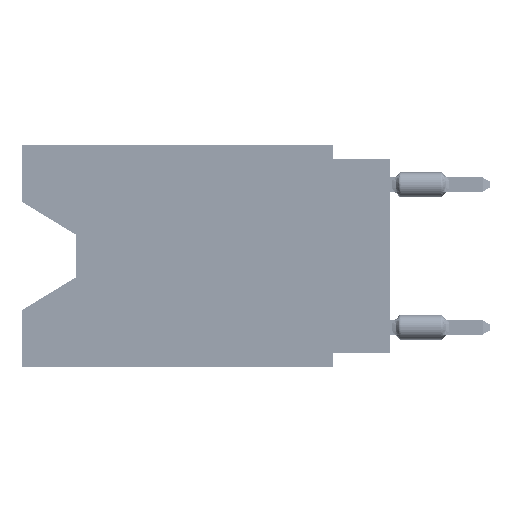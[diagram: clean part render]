
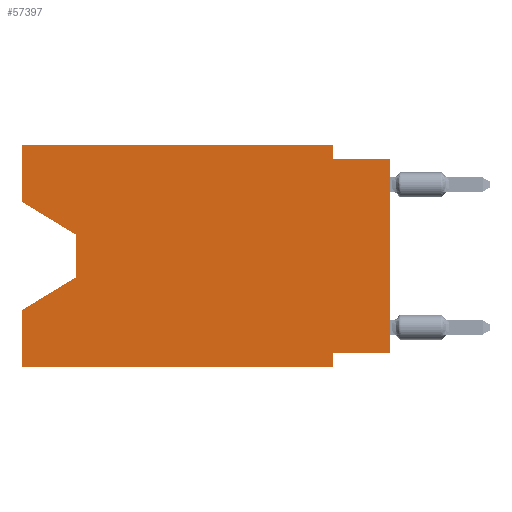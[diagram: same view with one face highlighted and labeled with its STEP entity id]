
A CAD part, left-side view. The second image highlights one B-rep face of the part: STEP entity #57397.
In plain terms, the highlighted planar face has unit normal (-1, 0, 0).
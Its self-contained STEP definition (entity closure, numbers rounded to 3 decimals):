
#237 = ORIENTED_EDGE ( 'NONE', *, *, #24268, .F. ) ;
#392 = LINE ( 'NONE', #14249, #2307 ) ;
#1442 = LINE ( 'NONE', #16250, #8433 ) ;
#2090 = CARTESIAN_POINT ( 'NONE',  ( 0., 16.383, -2.546 ) ) ;
#2156 = CARTESIAN_POINT ( 'NONE',  ( 0., 16.383, 0. ) ) ;
#2307 = VECTOR ( 'NONE', #44152, 1000. ) ;
#2761 = CARTESIAN_POINT ( 'NONE',  ( 0., 2.54, 0. ) ) ;
#2806 = DIRECTION ( 'NONE',  ( 0., -1., 0. ) ) ;
#3047 = CARTESIAN_POINT ( 'NONE',  ( 0., 0., 0. ) ) ;
#3791 = LINE ( 'NONE', #61402, #41108 ) ;
#5400 = LINE ( 'NONE', #29526, #29518 ) ;
#6170 = EDGE_CURVE ( 'NONE', #63260, #33809, #392, .T. ) ;
#6595 = VECTOR ( 'NONE', #26848, 1000. ) ;
#6658 = ORIENTED_EDGE ( 'NONE', *, *, #6170, .F. ) ;
#7143 = CARTESIAN_POINT ( 'NONE',  ( 0., 0., -9.271 ) ) ;
#7292 = DIRECTION ( 'NONE',  ( 0., 0., 1. ) ) ;
#8433 = VECTOR ( 'NONE', #35867, 1000. ) ;
#8668 = CARTESIAN_POINT ( 'NONE',  ( 0., 0., -0.635 ) ) ;
#9442 = CARTESIAN_POINT ( 'NONE',  ( 0., 2.54, -0.635 ) ) ;
#9578 = VECTOR ( 'NONE', #61229, 1000. ) ;
#10163 = EDGE_CURVE ( 'NONE', #46392, #38882, #5400, .T. ) ;
#11754 = LINE ( 'NONE', #2090, #62392 ) ;
#12866 = LINE ( 'NONE', #62095, #29187 ) ;
#13568 = DIRECTION ( 'NONE',  ( 0., 0., -1. ) ) ;
#13794 = VERTEX_POINT ( 'NONE', #39250 ) ;
#13812 = ORIENTED_EDGE ( 'NONE', *, *, #10163, .T. ) ;
#14249 = CARTESIAN_POINT ( 'NONE',  ( 0., 0., -0.635 ) ) ;
#16250 = CARTESIAN_POINT ( 'NONE',  ( 0., 13.97, -4.013 ) ) ;
#17311 = DIRECTION ( 'NONE',  ( 0., 0., -1. ) ) ;
#18388 = CARTESIAN_POINT ( 'NONE',  ( 0., 16.383, -2.546 ) ) ;
#18994 = CARTESIAN_POINT ( 'NONE',  ( 0., 16.383, 0. ) ) ;
#19054 = LINE ( 'NONE', #38683, #25056 ) ;
#19892 = CARTESIAN_POINT ( 'NONE',  ( 0., 16.383, -9.906 ) ) ;
#21064 = ORIENTED_EDGE ( 'NONE', *, *, #23473, .T. ) ;
#21758 = VERTEX_POINT ( 'NONE', #2761 ) ;
#22023 = DIRECTION ( 'NONE',  ( 0., -0.855, -0.519 ) ) ;
#22955 = ORIENTED_EDGE ( 'NONE', *, *, #55782, .F. ) ;
#23473 = EDGE_CURVE ( 'NONE', #36423, #37425, #11754, .T. ) ;
#24005 = CARTESIAN_POINT ( 'NONE',  ( 0., 13.97, -4.013 ) ) ;
#24205 = DIRECTION ( 'NONE',  ( 0., 0., 1. ) ) ;
#24268 = EDGE_CURVE ( 'NONE', #13794, #21758, #36276, .T. ) ;
#25056 = VECTOR ( 'NONE', #29040, 1000. ) ;
#26848 = DIRECTION ( 'NONE',  ( 0., 0., 1. ) ) ;
#27467 = ORIENTED_EDGE ( 'NONE', *, *, #28625, .T. ) ;
#28625 = EDGE_CURVE ( 'NONE', #37425, #46392, #1442, .T. ) ;
#29040 = DIRECTION ( 'NONE',  ( 0., -1., 0. ) ) ;
#29187 = VECTOR ( 'NONE', #33113, 1000. ) ;
#29518 = VECTOR ( 'NONE', #34356, 1000. ) ;
#29526 = CARTESIAN_POINT ( 'NONE',  ( 0., 13.97, -5.893 ) ) ;
#30471 = CARTESIAN_POINT ( 'NONE',  ( 0., 2.54, -9.271 ) ) ;
#31993 = VERTEX_POINT ( 'NONE', #7143 ) ;
#32337 = CARTESIAN_POINT ( 'NONE',  ( 0., 16.383, -7.36 ) ) ;
#32548 = ORIENTED_EDGE ( 'NONE', *, *, #59931, .F. ) ;
#33113 = DIRECTION ( 'NONE',  ( 0., 0., -1. ) ) ;
#33809 = VERTEX_POINT ( 'NONE', #8668 ) ;
#34129 = PLANE ( 'NONE',  #60729 ) ;
#34356 = DIRECTION ( 'NONE',  ( 0., 0.855, -0.519 ) ) ;
#35867 = DIRECTION ( 'NONE',  ( 0., 0., -1. ) ) ;
#36276 = LINE ( 'NONE', #50768, #47021 ) ;
#36423 = VERTEX_POINT ( 'NONE', #18388 ) ;
#37425 = VERTEX_POINT ( 'NONE', #24005 ) ;
#37687 = DIRECTION ( 'NONE',  ( 1., 0., 0. ) ) ;
#38162 = VECTOR ( 'NONE', #7292, 1000. ) ;
#38683 = CARTESIAN_POINT ( 'NONE',  ( 0., 16.383, -9.906 ) ) ;
#38882 = VERTEX_POINT ( 'NONE', #32337 ) ;
#39250 = CARTESIAN_POINT ( 'NONE',  ( 0., 16.383, 0. ) ) ;
#39667 = EDGE_LOOP ( 'NONE', ( #21064, #27467, #13812, #22955, #42672, #58828, #32548, #61597, #6658, #39751, #237, #48209 ) ) ;
#39751 = ORIENTED_EDGE ( 'NONE', *, *, #53253, .F. ) ;
#41085 = LINE ( 'NONE', #2156, #38162 ) ;
#41108 = VECTOR ( 'NONE', #17311, 1000. ) ;
#42329 = EDGE_CURVE ( 'NONE', #53451, #61373, #12866, .T. ) ;
#42672 = ORIENTED_EDGE ( 'NONE', *, *, #62521, .T. ) ;
#43158 = EDGE_CURVE ( 'NONE', #31993, #33809, #50988, .T. ) ;
#43221 = LINE ( 'NONE', #47732, #60589 ) ;
#44152 = DIRECTION ( 'NONE',  ( 0., -1., 0. ) ) ;
#46098 = CARTESIAN_POINT ( 'NONE',  ( 0., 0., -9.271 ) ) ;
#46392 = VERTEX_POINT ( 'NONE', #49923 ) ;
#47021 = VECTOR ( 'NONE', #2806, 1000. ) ;
#47732 = CARTESIAN_POINT ( 'NONE',  ( 0., 16.383, 0. ) ) ;
#48027 = CARTESIAN_POINT ( 'NONE',  ( 0., 2.54, -9.906 ) ) ;
#48209 = ORIENTED_EDGE ( 'NONE', *, *, #58061, .F. ) ;
#49923 = CARTESIAN_POINT ( 'NONE',  ( 0., 13.97, -5.893 ) ) ;
#50768 = CARTESIAN_POINT ( 'NONE',  ( 0., 16.383, 0. ) ) ;
#50988 = LINE ( 'NONE', #3047, #6595 ) ;
#53253 = EDGE_CURVE ( 'NONE', #21758, #63260, #3791, .T. ) ;
#53451 = VERTEX_POINT ( 'NONE', #30471 ) ;
#55131 = LINE ( 'NONE', #46098, #9578 ) ;
#55782 = EDGE_CURVE ( 'NONE', #58890, #38882, #43221, .T. ) ;
#57397 = ADVANCED_FACE ( 'NONE', ( #62164 ), #34129, .F. ) ;
#58061 = EDGE_CURVE ( 'NONE', #36423, #13794, #41085, .T. ) ;
#58828 = ORIENTED_EDGE ( 'NONE', *, *, #42329, .F. ) ;
#58890 = VERTEX_POINT ( 'NONE', #19892 ) ;
#59931 = EDGE_CURVE ( 'NONE', #31993, #53451, #55131, .T. ) ;
#60589 = VECTOR ( 'NONE', #24205, 1000. ) ;
#60729 = AXIS2_PLACEMENT_3D ( 'NONE', #18994, #37687, #13568 ) ;
#61229 = DIRECTION ( 'NONE',  ( 0., 1., 0. ) ) ;
#61373 = VERTEX_POINT ( 'NONE', #48027 ) ;
#61402 = CARTESIAN_POINT ( 'NONE',  ( 0., 2.54, 0. ) ) ;
#61597 = ORIENTED_EDGE ( 'NONE', *, *, #43158, .T. ) ;
#62095 = CARTESIAN_POINT ( 'NONE',  ( 0., 2.54, -9.906 ) ) ;
#62164 = FACE_OUTER_BOUND ( 'NONE', #39667, .T. ) ;
#62392 = VECTOR ( 'NONE', #22023, 1000. ) ;
#62521 = EDGE_CURVE ( 'NONE', #58890, #61373, #19054, .T. ) ;
#63260 = VERTEX_POINT ( 'NONE', #9442 ) ;
